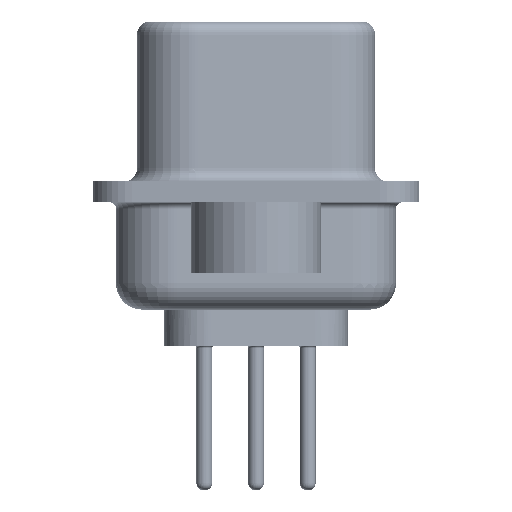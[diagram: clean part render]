
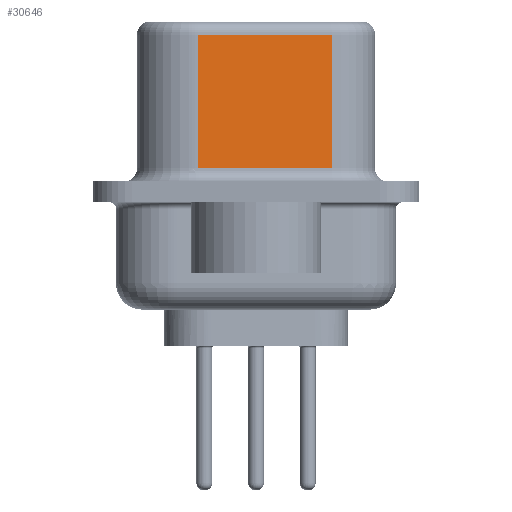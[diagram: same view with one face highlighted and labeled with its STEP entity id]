
A CAD part, left-side view. The second image highlights one B-rep face of the part: STEP entity #30646.
In plain terms, the highlighted planar face has unit normal (-0.985, -0.174, 0).
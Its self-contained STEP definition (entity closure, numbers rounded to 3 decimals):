
#1230 = CARTESIAN_POINT ( 'NONE',  ( 4.58, -2.897, 6.02 ) ) ;
#4537 = VERTEX_POINT ( 'NONE', #24126 ) ;
#4939 = EDGE_LOOP ( 'NONE', ( #12601, #15012, #6958, #19850 ) ) ;
#5570 = CARTESIAN_POINT ( 'NONE',  ( 4.58, -2.897, 6.52 ) ) ;
#6958 = ORIENTED_EDGE ( 'NONE', *, *, #14519, .T. ) ;
#7524 = VECTOR ( 'NONE', #32505, 1000. ) ;
#7785 = LINE ( 'NONE', #8455, #13739 ) ;
#8124 = DIRECTION ( 'NONE',  ( -0.174, 0.985, 0. ) ) ;
#8455 = CARTESIAN_POINT ( 'NONE',  ( 4.58, -2.897, 6.02 ) ) ;
#8474 = VERTEX_POINT ( 'NONE', #10093 ) ;
#10093 = CARTESIAN_POINT ( 'NONE',  ( 3.68, 2.203, 0.9 ) ) ;
#10318 = LINE ( 'NONE', #28247, #12669 ) ;
#10782 = DIRECTION ( 'NONE',  ( 0., 0., -1. ) ) ;
#12601 = ORIENTED_EDGE ( 'NONE', *, *, #17725, .F. ) ;
#12669 = VECTOR ( 'NONE', #10782, 1000. ) ;
#13479 = VECTOR ( 'NONE', #28888, 1000. ) ;
#13608 = AXIS2_PLACEMENT_3D ( 'NONE', #5570, #23169, #8124 ) ;
#13739 = VECTOR ( 'NONE', #28363, 1000. ) ;
#14008 = VERTEX_POINT ( 'NONE', #1230 ) ;
#14371 = EDGE_CURVE ( 'NONE', #8474, #4537, #28303, .T. ) ;
#14519 = EDGE_CURVE ( 'NONE', #32039, #8474, #10318, .T. ) ;
#14741 = FACE_OUTER_BOUND ( 'NONE', #4939, .T. ) ;
#15012 = ORIENTED_EDGE ( 'NONE', *, *, #17580, .T. ) ;
#17580 = EDGE_CURVE ( 'NONE', #14008, #32039, #7785, .T. ) ;
#17718 = CARTESIAN_POINT ( 'NONE',  ( 4.58, -2.897, 0.9 ) ) ;
#17725 = EDGE_CURVE ( 'NONE', #14008, #4537, #26779, .T. ) ;
#19850 = ORIENTED_EDGE ( 'NONE', *, *, #14371, .T. ) ;
#20647 = PLANE ( 'NONE',  #13608 ) ;
#21527 = CARTESIAN_POINT ( 'NONE',  ( 4.58, -2.897, 6.52 ) ) ;
#23169 = DIRECTION ( 'NONE',  ( 0.985, 0.174, 0. ) ) ;
#24126 = CARTESIAN_POINT ( 'NONE',  ( 4.58, -2.897, 0.9 ) ) ;
#26779 = LINE ( 'NONE', #21527, #13479 ) ;
#28247 = CARTESIAN_POINT ( 'NONE',  ( 3.68, 2.203, 6.52 ) ) ;
#28303 = LINE ( 'NONE', #17718, #7524 ) ;
#28363 = DIRECTION ( 'NONE',  ( -0.174, 0.985, 0. ) ) ;
#28888 = DIRECTION ( 'NONE',  ( 0., 0., -1. ) ) ;
#30646 = ADVANCED_FACE ( 'NONE', ( #14741 ), #20647, .F. ) ;
#31643 = CARTESIAN_POINT ( 'NONE',  ( 3.68, 2.203, 6.02 ) ) ;
#32039 = VERTEX_POINT ( 'NONE', #31643 ) ;
#32505 = DIRECTION ( 'NONE',  ( 0.174, -0.985, 0. ) ) ;
